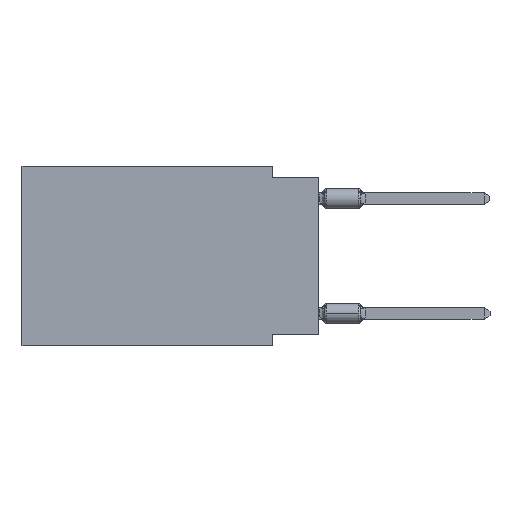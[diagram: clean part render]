
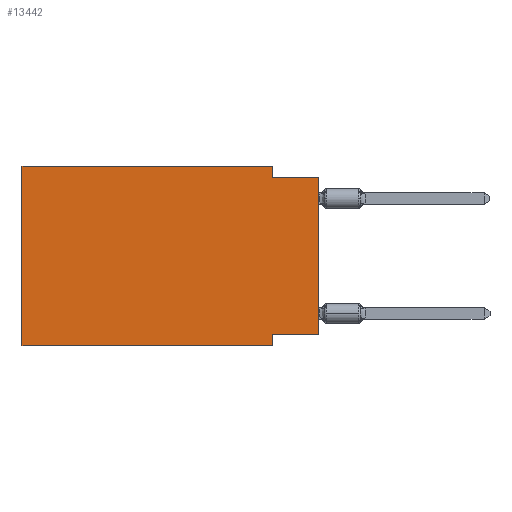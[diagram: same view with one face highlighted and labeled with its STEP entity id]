
A CAD part, left-side view. The second image highlights one B-rep face of the part: STEP entity #13442.
In plain terms, the highlighted planar face has unit normal (-1, 0, 0).
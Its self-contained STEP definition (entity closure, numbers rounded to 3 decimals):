
#328 = DIRECTION ( 'NONE',  ( 0., -1., 0. ) ) ;
#572 = CARTESIAN_POINT ( 'NONE',  ( 0., 16.383, 0. ) ) ;
#791 = EDGE_CURVE ( 'NONE', #8039, #3752, #15021, .T. ) ;
#1363 = VECTOR ( 'NONE', #328, 1000. ) ;
#1414 = VERTEX_POINT ( 'NONE', #11583 ) ;
#1566 = EDGE_CURVE ( 'NONE', #15988, #4740, #8352, .T. ) ;
#2005 = DIRECTION ( 'NONE',  ( 1., 0., 0. ) ) ;
#2531 = VERTEX_POINT ( 'NONE', #4566 ) ;
#2763 = CARTESIAN_POINT ( 'NONE',  ( 0., 2.54, -9.271 ) ) ;
#3244 = VECTOR ( 'NONE', #11762, 1000. ) ;
#3485 = VERTEX_POINT ( 'NONE', #5908 ) ;
#3707 = VECTOR ( 'NONE', #11263, 1000. ) ;
#3752 = VERTEX_POINT ( 'NONE', #2763 ) ;
#3793 = ORIENTED_EDGE ( 'NONE', *, *, #12522, .T. ) ;
#4377 = CARTESIAN_POINT ( 'NONE',  ( 0., 16.383, 0. ) ) ;
#4543 = CARTESIAN_POINT ( 'NONE',  ( 0., 2.54, 0. ) ) ;
#4566 = CARTESIAN_POINT ( 'NONE',  ( 0., 2.54, 0. ) ) ;
#4719 = PLANE ( 'NONE',  #12411 ) ;
#4740 = VERTEX_POINT ( 'NONE', #5997 ) ;
#4884 = DIRECTION ( 'NONE',  ( 0., 0., 1. ) ) ;
#5164 = CARTESIAN_POINT ( 'NONE',  ( 0., 2.54, -9.906 ) ) ;
#5196 = ORIENTED_EDGE ( 'NONE', *, *, #13991, .F. ) ;
#5719 = ORIENTED_EDGE ( 'NONE', *, *, #1566, .F. ) ;
#5843 = EDGE_LOOP ( 'NONE', ( #13090, #5196, #16611, #11121, #5719, #3793, #8405, #8257 ) ) ;
#5908 = CARTESIAN_POINT ( 'NONE',  ( 0., 2.54, -9.906 ) ) ;
#5997 = CARTESIAN_POINT ( 'NONE',  ( 0., 16.383, 0. ) ) ;
#6006 = LINE ( 'NONE', #4543, #8077 ) ;
#6097 = CARTESIAN_POINT ( 'NONE',  ( 0., 0., 0. ) ) ;
#6886 = EDGE_CURVE ( 'NONE', #4740, #2531, #8648, .T. ) ;
#6940 = CARTESIAN_POINT ( 'NONE',  ( 0., 16.383, -9.906 ) ) ;
#7840 = LINE ( 'NONE', #5164, #3244 ) ;
#8039 = VERTEX_POINT ( 'NONE', #11388 ) ;
#8077 = VECTOR ( 'NONE', #12534, 1000. ) ;
#8110 = EDGE_CURVE ( 'NONE', #2531, #10466, #6006, .T. ) ;
#8128 = DIRECTION ( 'NONE',  ( 0., -1., 0. ) ) ;
#8257 = ORIENTED_EDGE ( 'NONE', *, *, #791, .F. ) ;
#8272 = DIRECTION ( 'NONE',  ( 0., 0., 1. ) ) ;
#8352 = LINE ( 'NONE', #4377, #11492 ) ;
#8395 = CARTESIAN_POINT ( 'NONE',  ( 0., 0., -9.271 ) ) ;
#8405 = ORIENTED_EDGE ( 'NONE', *, *, #10182, .F. ) ;
#8648 = LINE ( 'NONE', #572, #9986 ) ;
#9434 = CARTESIAN_POINT ( 'NONE',  ( 0., 16.383, -9.906 ) ) ;
#9986 = VECTOR ( 'NONE', #13730, 1000. ) ;
#10182 = EDGE_CURVE ( 'NONE', #3752, #3485, #7840, .T. ) ;
#10347 = CARTESIAN_POINT ( 'NONE',  ( 0., 2.54, -0.635 ) ) ;
#10466 = VERTEX_POINT ( 'NONE', #10347 ) ;
#11121 = ORIENTED_EDGE ( 'NONE', *, *, #6886, .F. ) ;
#11263 = DIRECTION ( 'NONE',  ( 0., 1., 0. ) ) ;
#11388 = CARTESIAN_POINT ( 'NONE',  ( 0., 0., -9.271 ) ) ;
#11492 = VECTOR ( 'NONE', #8272, 1000. ) ;
#11583 = CARTESIAN_POINT ( 'NONE',  ( 0., 0., -0.635 ) ) ;
#11762 = DIRECTION ( 'NONE',  ( 0., 0., -1. ) ) ;
#12411 = AXIS2_PLACEMENT_3D ( 'NONE', #13949, #2005, #16774 ) ;
#12522 = EDGE_CURVE ( 'NONE', #15988, #3485, #16149, .T. ) ;
#12534 = DIRECTION ( 'NONE',  ( 0., 0., -1. ) ) ;
#12625 = LINE ( 'NONE', #6097, #15451 ) ;
#12970 = VECTOR ( 'NONE', #8128, 1000. ) ;
#13090 = ORIENTED_EDGE ( 'NONE', *, *, #13371, .T. ) ;
#13120 = LINE ( 'NONE', #14594, #12970 ) ;
#13371 = EDGE_CURVE ( 'NONE', #8039, #1414, #12625, .T. ) ;
#13442 = ADVANCED_FACE ( 'NONE', ( #15330 ), #4719, .F. ) ;
#13730 = DIRECTION ( 'NONE',  ( 0., -1., 0. ) ) ;
#13949 = CARTESIAN_POINT ( 'NONE',  ( 0., 16.383, 0. ) ) ;
#13991 = EDGE_CURVE ( 'NONE', #10466, #1414, #13120, .T. ) ;
#14594 = CARTESIAN_POINT ( 'NONE',  ( 0., 0., -0.635 ) ) ;
#15021 = LINE ( 'NONE', #8395, #3707 ) ;
#15330 = FACE_OUTER_BOUND ( 'NONE', #5843, .T. ) ;
#15451 = VECTOR ( 'NONE', #4884, 1000. ) ;
#15988 = VERTEX_POINT ( 'NONE', #9434 ) ;
#16149 = LINE ( 'NONE', #6940, #1363 ) ;
#16611 = ORIENTED_EDGE ( 'NONE', *, *, #8110, .F. ) ;
#16774 = DIRECTION ( 'NONE',  ( 0., 0., -1. ) ) ;
